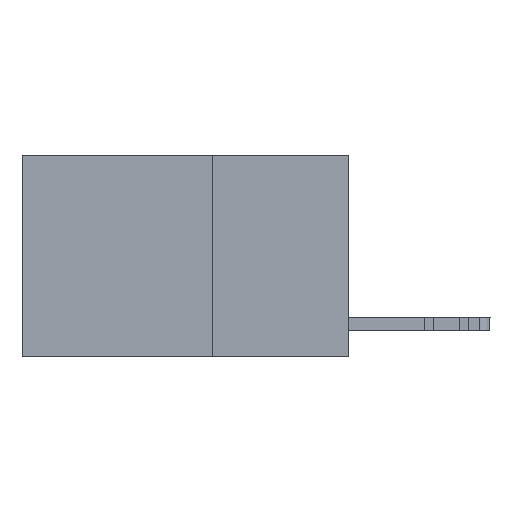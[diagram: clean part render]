
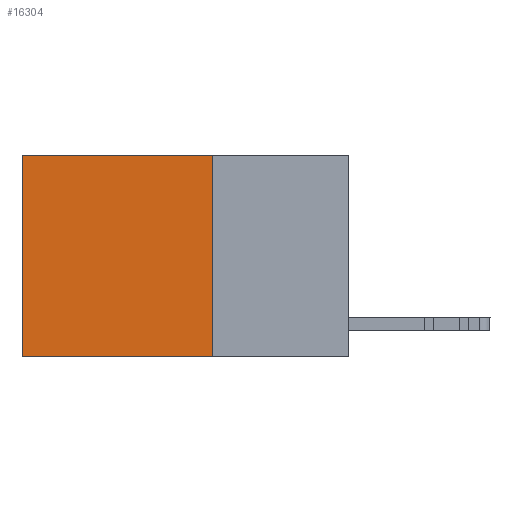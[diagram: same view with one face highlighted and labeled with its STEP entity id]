
A CAD part, left-side view. The second image highlights one B-rep face of the part: STEP entity #16304.
In plain terms, the highlighted planar face has unit normal (-1, 0, 0).
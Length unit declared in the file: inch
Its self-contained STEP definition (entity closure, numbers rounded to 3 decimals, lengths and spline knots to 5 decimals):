
#1187 = VERTEX_POINT ( 'NONE', #24749 ) ;
#1327 = ORIENTED_EDGE ( 'NONE', *, *, #21505, .T. ) ;
#1336 = FACE_OUTER_BOUND ( 'NONE', #13925, .T. ) ;
#1528 = CARTESIAN_POINT ( 'NONE',  ( 0.2625, 0.25, 0. ) ) ;
#1587 = CARTESIAN_POINT ( 'NONE',  ( 0.2625, 0.25, 0. ) ) ;
#3626 = LINE ( 'NONE', #8573, #14962 ) ;
#3864 = DIRECTION ( 'NONE',  ( 0., 1., 0. ) ) ;
#3990 = CARTESIAN_POINT ( 'NONE',  ( 0.2625, 0.25, -0.37 ) ) ;
#4018 = VERTEX_POINT ( 'NONE', #3990 ) ;
#4677 = EDGE_CURVE ( 'NONE', #10355, #4018, #3626, .T. ) ;
#5558 = ORIENTED_EDGE ( 'NONE', *, *, #14782, .T. ) ;
#5950 = EDGE_CURVE ( 'NONE', #4018, #12724, #7876, .T. ) ;
#6982 = CARTESIAN_POINT ( 'NONE',  ( 0.2625, 0.6, -0.37 ) ) ;
#7648 = CARTESIAN_POINT ( 'NONE',  ( 0.2625, 0.6, 0. ) ) ;
#7876 = LINE ( 'NONE', #15375, #18979 ) ;
#7953 = VECTOR ( 'NONE', #18710, 39.37008 ) ;
#8573 = CARTESIAN_POINT ( 'NONE',  ( 0.2625, 0.25, 0. ) ) ;
#8682 = LINE ( 'NONE', #7648, #7953 ) ;
#10355 = VERTEX_POINT ( 'NONE', #12761 ) ;
#10822 = DIRECTION ( 'NONE',  ( 0., 0., -1. ) ) ;
#10849 = DIRECTION ( 'NONE',  ( 0., 0., -1. ) ) ;
#12724 = VERTEX_POINT ( 'NONE', #6982 ) ;
#12761 = CARTESIAN_POINT ( 'NONE',  ( 0.2625, 0.25, 0. ) ) ;
#13168 = DIRECTION ( 'NONE',  ( 0., 1., 0. ) ) ;
#13925 = EDGE_LOOP ( 'NONE', ( #5558, #24132, #28555, #1327 ) ) ;
#14574 = LINE ( 'NONE', #1528, #25491 ) ;
#14782 = EDGE_CURVE ( 'NONE', #1187, #12724, #8682, .T. ) ;
#14962 = VECTOR ( 'NONE', #10849, 39.37008 ) ;
#15375 = CARTESIAN_POINT ( 'NONE',  ( 0.2625, 0.25, -0.37 ) ) ;
#16304 = ADVANCED_FACE ( 'NONE', ( #1336 ), #21767, .F. ) ;
#18710 = DIRECTION ( 'NONE',  ( 0., 0., -1. ) ) ;
#18979 = VECTOR ( 'NONE', #13168, 39.37008 ) ;
#19292 = AXIS2_PLACEMENT_3D ( 'NONE', #1587, #23959, #10822 ) ;
#21505 = EDGE_CURVE ( 'NONE', #10355, #1187, #14574, .T. ) ;
#21767 = PLANE ( 'NONE',  #19292 ) ;
#23959 = DIRECTION ( 'NONE',  ( 1., 0., 0. ) ) ;
#24132 = ORIENTED_EDGE ( 'NONE', *, *, #5950, .F. ) ;
#24749 = CARTESIAN_POINT ( 'NONE',  ( 0.2625, 0.6, 0. ) ) ;
#25491 = VECTOR ( 'NONE', #3864, 39.37008 ) ;
#28555 = ORIENTED_EDGE ( 'NONE', *, *, #4677, .F. ) ;
